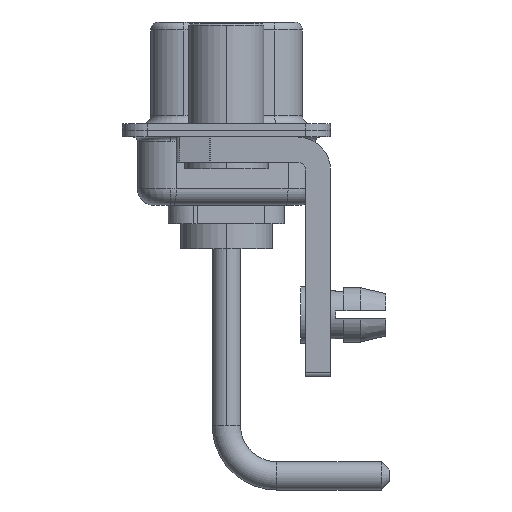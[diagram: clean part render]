
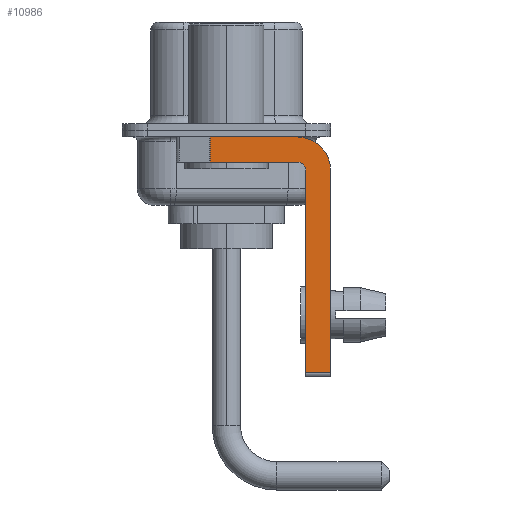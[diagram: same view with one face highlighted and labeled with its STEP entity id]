
A CAD part, left-side view. The second image highlights one B-rep face of the part: STEP entity #10986.
In plain terms, the highlighted planar face has unit normal (-1, 0, 0).
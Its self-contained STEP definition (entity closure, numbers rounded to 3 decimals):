
#161 = VERTEX_POINT ( 'NONE', #13061 ) ;
#185 = DIRECTION ( 'NONE',  ( 1., 0., 0. ) ) ;
#376 = LINE ( 'NONE', #5927, #1842 ) ;
#405 = CARTESIAN_POINT ( 'NONE',  ( -2.9, 0.978, -1.9 ) ) ;
#1490 = CIRCLE ( 'NONE', #5853, 2. ) ;
#1842 = VECTOR ( 'NONE', #11467, 1000. ) ;
#1885 = ORIENTED_EDGE ( 'NONE', *, *, #7375, .F. ) ;
#2202 = DIRECTION ( 'NONE',  ( 1., 0., 0. ) ) ;
#2913 = VECTOR ( 'NONE', #15691, 1000. ) ;
#2925 = VECTOR ( 'NONE', #14391, 1000. ) ;
#3191 = ORIENTED_EDGE ( 'NONE', *, *, #4874, .F. ) ;
#3478 = LINE ( 'NONE', #405, #2925 ) ;
#3613 = CARTESIAN_POINT ( 'NONE',  ( -2.9, -4.25, -0.4 ) ) ;
#4266 = VERTEX_POINT ( 'NONE', #4496 ) ;
#4357 = DIRECTION ( 'NONE',  ( 0., 0., -1. ) ) ;
#4496 = CARTESIAN_POINT ( 'NONE',  ( -2.9, 0.978, -0.4 ) ) ;
#4740 = DIRECTION ( 'NONE',  ( 0., -1., 0. ) ) ;
#4835 = EDGE_CURVE ( 'NONE', #17846, #6783, #1490, .T. ) ;
#4874 = EDGE_CURVE ( 'NONE', #6783, #11742, #5649, .T. ) ;
#5464 = VERTEX_POINT ( 'NONE', #17541 ) ;
#5649 = LINE ( 'NONE', #15337, #15401 ) ;
#5853 = AXIS2_PLACEMENT_3D ( 'NONE', #8635, #185, #4357 ) ;
#5889 = VERTEX_POINT ( 'NONE', #17428 ) ;
#5927 = CARTESIAN_POINT ( 'NONE',  ( -2.9, -4.75, -14.8 ) ) ;
#6028 = EDGE_CURVE ( 'NONE', #161, #11742, #6109, .T. ) ;
#6044 = DIRECTION ( 'NONE',  ( -1., 0., 0. ) ) ;
#6066 = CARTESIAN_POINT ( 'NONE',  ( -2.9, -4.25, -1.9 ) ) ;
#6109 = LINE ( 'NONE', #17176, #15400 ) ;
#6783 = VERTEX_POINT ( 'NONE', #14507 ) ;
#6859 = VERTEX_POINT ( 'NONE', #6066 ) ;
#7258 = EDGE_LOOP ( 'NONE', ( #14049, #17942, #12344, #1885, #12309, #8211, #3191, #12969 ) ) ;
#7375 = EDGE_CURVE ( 'NONE', #5464, #6859, #16349, .T. ) ;
#8211 = ORIENTED_EDGE ( 'NONE', *, *, #6028, .T. ) ;
#8635 = CARTESIAN_POINT ( 'NONE',  ( -2.9, -4.25, -2.4 ) ) ;
#10166 = LINE ( 'NONE', #14072, #2913 ) ;
#10229 = CARTESIAN_POINT ( 'NONE',  ( -2.9, -6.25, -14.55 ) ) ;
#10489 = VECTOR ( 'NONE', #12425, 1000. ) ;
#10986 = ADVANCED_FACE ( 'NONE', ( #16167 ), #13539, .F. ) ;
#11467 = DIRECTION ( 'NONE',  ( 0., 0., 1. ) ) ;
#11723 = AXIS2_PLACEMENT_3D ( 'NONE', #13116, #6044, #11760 ) ;
#11742 = VERTEX_POINT ( 'NONE', #10229 ) ;
#11760 = DIRECTION ( 'NONE',  ( 0., 0., 1. ) ) ;
#12089 = DIRECTION ( 'NONE',  ( 0., 0., -1. ) ) ;
#12309 = ORIENTED_EDGE ( 'NONE', *, *, #16099, .F. ) ;
#12344 = ORIENTED_EDGE ( 'NONE', *, *, #13109, .F. ) ;
#12425 = DIRECTION ( 'NONE',  ( 0., -1., 0. ) ) ;
#12615 = LINE ( 'NONE', #16777, #10489 ) ;
#12969 = ORIENTED_EDGE ( 'NONE', *, *, #4835, .F. ) ;
#13026 = AXIS2_PLACEMENT_3D ( 'NONE', #13453, #2202, #12089 ) ;
#13061 = CARTESIAN_POINT ( 'NONE',  ( -2.9, -4.75, -14.55 ) ) ;
#13109 = EDGE_CURVE ( 'NONE', #6859, #5889, #10166, .T. ) ;
#13116 = CARTESIAN_POINT ( 'NONE',  ( -2.9, -4.25, -2.4 ) ) ;
#13453 = CARTESIAN_POINT ( 'NONE',  ( -2.9, -4.25, -2.4 ) ) ;
#13539 = PLANE ( 'NONE',  #13026 ) ;
#13568 = EDGE_CURVE ( 'NONE', #4266, #5889, #3478, .T. ) ;
#14049 = ORIENTED_EDGE ( 'NONE', *, *, #14285, .F. ) ;
#14072 = CARTESIAN_POINT ( 'NONE',  ( -2.9, -4.25, -1.9 ) ) ;
#14285 = EDGE_CURVE ( 'NONE', #4266, #17846, #12615, .T. ) ;
#14391 = DIRECTION ( 'NONE',  ( 0., 0., -1. ) ) ;
#14507 = CARTESIAN_POINT ( 'NONE',  ( -2.9, -6.25, -2.4 ) ) ;
#15337 = CARTESIAN_POINT ( 'NONE',  ( -2.9, -6.25, -2.4 ) ) ;
#15400 = VECTOR ( 'NONE', #4740, 1000. ) ;
#15401 = VECTOR ( 'NONE', #15434, 1000. ) ;
#15434 = DIRECTION ( 'NONE',  ( 0., 0., -1. ) ) ;
#15691 = DIRECTION ( 'NONE',  ( 0., 1., 0. ) ) ;
#16099 = EDGE_CURVE ( 'NONE', #161, #5464, #376, .T. ) ;
#16167 = FACE_OUTER_BOUND ( 'NONE', #7258, .T. ) ;
#16349 = CIRCLE ( 'NONE', #11723, 0.5 ) ;
#16777 = CARTESIAN_POINT ( 'NONE',  ( -2.9, 3., -0.4 ) ) ;
#17176 = CARTESIAN_POINT ( 'NONE',  ( -2.9, -4.25, -14.55 ) ) ;
#17428 = CARTESIAN_POINT ( 'NONE',  ( -2.9, 0.978, -1.9 ) ) ;
#17541 = CARTESIAN_POINT ( 'NONE',  ( -2.9, -4.75, -2.4 ) ) ;
#17846 = VERTEX_POINT ( 'NONE', #3613 ) ;
#17942 = ORIENTED_EDGE ( 'NONE', *, *, #13568, .T. ) ;
